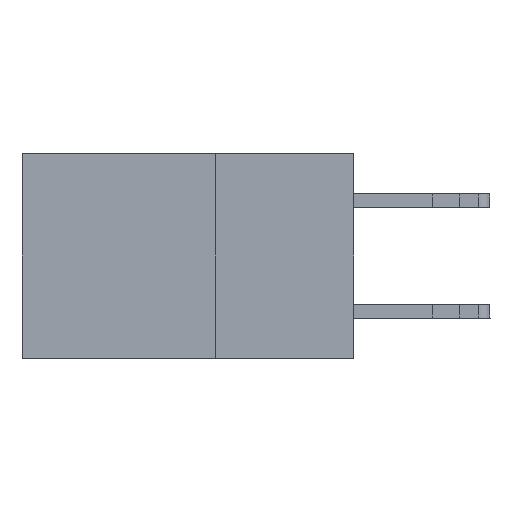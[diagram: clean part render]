
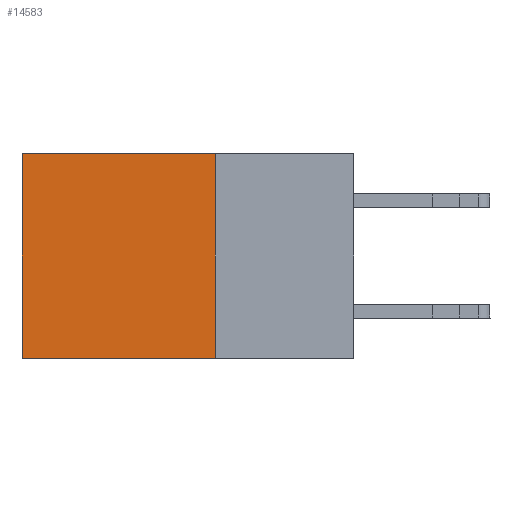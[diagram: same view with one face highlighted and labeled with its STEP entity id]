
A CAD part, left-side view. The second image highlights one B-rep face of the part: STEP entity #14583.
In plain terms, the highlighted planar face has unit normal (-1, 0, 0).
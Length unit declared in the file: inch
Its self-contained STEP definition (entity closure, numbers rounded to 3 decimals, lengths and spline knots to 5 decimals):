
#366 = CARTESIAN_POINT ( 'NONE',  ( 0.2875, 0.6, -0.37 ) ) ;
#434 = VERTEX_POINT ( 'NONE', #3841 ) ;
#848 = CARTESIAN_POINT ( 'NONE',  ( 0.2875, 0.25, -0.37 ) ) ;
#1038 = CARTESIAN_POINT ( 'NONE',  ( 0.2875, 0.25, -0.37 ) ) ;
#3162 = EDGE_CURVE ( 'NONE', #11246, #14346, #31906, .T. ) ;
#3841 = CARTESIAN_POINT ( 'NONE',  ( 0.2875, 0.6, 0. ) ) ;
#4892 = CARTESIAN_POINT ( 'NONE',  ( 0.2875, 0.25, 0. ) ) ;
#6166 = EDGE_CURVE ( 'NONE', #29661, #11246, #13900, .T. ) ;
#6251 = VECTOR ( 'NONE', #19085, 39.37008 ) ;
#8192 = EDGE_CURVE ( 'NONE', #29661, #434, #23126, .T. ) ;
#9456 = DIRECTION ( 'NONE',  ( 0., 0., -1. ) ) ;
#10428 = VECTOR ( 'NONE', #31950, 39.37008 ) ;
#10992 = EDGE_CURVE ( 'NONE', #434, #14346, #13581, .T. ) ;
#11054 = CARTESIAN_POINT ( 'NONE',  ( 0.2875, 0.6, 0. ) ) ;
#11246 = VERTEX_POINT ( 'NONE', #848 ) ;
#13581 = LINE ( 'NONE', #11054, #21346 ) ;
#13900 = LINE ( 'NONE', #29752, #10428 ) ;
#14346 = VERTEX_POINT ( 'NONE', #366 ) ;
#14583 = ADVANCED_FACE ( 'NONE', ( #17376 ), #20409, .F. ) ;
#16778 = CARTESIAN_POINT ( 'NONE',  ( 0.2875, 0.25, 0. ) ) ;
#17376 = FACE_OUTER_BOUND ( 'NONE', #18344, .T. ) ;
#18344 = EDGE_LOOP ( 'NONE', ( #24343, #30409, #24073, #29144 ) ) ;
#19085 = DIRECTION ( 'NONE',  ( 0., 1., 0. ) ) ;
#20409 = PLANE ( 'NONE',  #26277 ) ;
#20414 = DIRECTION ( 'NONE',  ( 0., 1., 0. ) ) ;
#20577 = CARTESIAN_POINT ( 'NONE',  ( 0.2875, 0.25, 0. ) ) ;
#21346 = VECTOR ( 'NONE', #21347, 39.37008 ) ;
#21347 = DIRECTION ( 'NONE',  ( 0., 0., -1. ) ) ;
#23126 = LINE ( 'NONE', #20577, #25537 ) ;
#24073 = ORIENTED_EDGE ( 'NONE', *, *, #6166, .F. ) ;
#24343 = ORIENTED_EDGE ( 'NONE', *, *, #10992, .T. ) ;
#25537 = VECTOR ( 'NONE', #20414, 39.37008 ) ;
#26277 = AXIS2_PLACEMENT_3D ( 'NONE', #4892, #27677, #9456 ) ;
#27677 = DIRECTION ( 'NONE',  ( 1., 0., 0. ) ) ;
#29144 = ORIENTED_EDGE ( 'NONE', *, *, #8192, .T. ) ;
#29661 = VERTEX_POINT ( 'NONE', #16778 ) ;
#29752 = CARTESIAN_POINT ( 'NONE',  ( 0.2875, 0.25, 0. ) ) ;
#30409 = ORIENTED_EDGE ( 'NONE', *, *, #3162, .F. ) ;
#31906 = LINE ( 'NONE', #1038, #6251 ) ;
#31950 = DIRECTION ( 'NONE',  ( 0., 0., -1. ) ) ;
